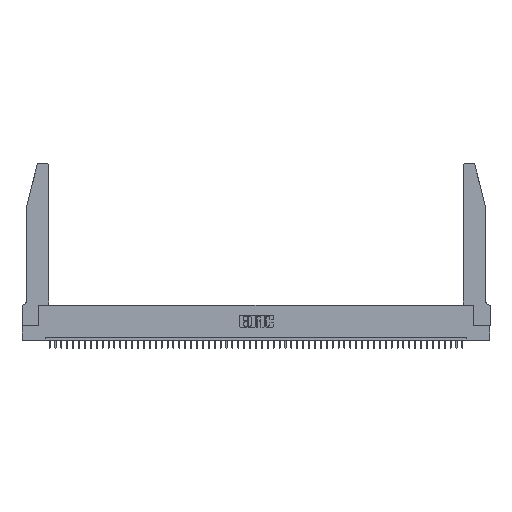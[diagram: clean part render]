
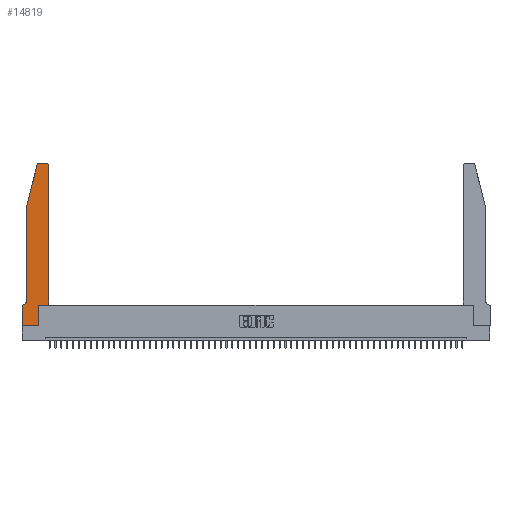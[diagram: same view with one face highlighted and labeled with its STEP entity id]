
A CAD part, top view. The second image highlights one B-rep face of the part: STEP entity #14819.
In plain terms, the highlighted planar face has unit normal (0, 0, 1).
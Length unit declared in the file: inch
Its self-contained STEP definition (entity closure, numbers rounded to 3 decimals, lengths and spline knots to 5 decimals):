
#916 = CIRCLE ( 'NONE', #51870, 0.07 ) ;
#919 = CARTESIAN_POINT ( 'NONE',  ( 0.0755, 2., 0.37 ) ) ;
#933 = DIRECTION ( 'NONE',  ( -1., 0., 0. ) ) ;
#1855 = VERTEX_POINT ( 'NONE', #25983 ) ;
#2791 = DIRECTION ( 'NONE',  ( -1., 0., 0. ) ) ;
#3752 = CARTESIAN_POINT ( 'NONE',  ( 0.2865, 0.35, 0.37 ) ) ;
#4103 = VECTOR ( 'NONE', #9275, 39.37008 ) ;
#4312 = EDGE_CURVE ( 'NONE', #38488, #1855, #916, .T. ) ;
#4542 = EDGE_LOOP ( 'NONE', ( #33524, #12257, #28069, #42367, #4695, #42255, #17631, #28983, #12638, #35962, #44566, #4682 ) ) ;
#4682 = ORIENTED_EDGE ( 'NONE', *, *, #17564, .T. ) ;
#4695 = ORIENTED_EDGE ( 'NONE', *, *, #4312, .T. ) ;
#5327 = LINE ( 'NONE', #21493, #29639 ) ;
#5565 = EDGE_CURVE ( 'NONE', #1855, #5975, #53952, .T. ) ;
#5975 = VERTEX_POINT ( 'NONE', #29071 ) ;
#6150 = VERTEX_POINT ( 'NONE', #25488 ) ;
#6459 = DIRECTION ( 'NONE',  ( 0., 0., 1. ) ) ;
#7187 = DIRECTION ( 'NONE',  ( -1., 0., 0. ) ) ;
#7304 = VERTEX_POINT ( 'NONE', #8736 ) ;
#7471 = CARTESIAN_POINT ( 'NONE',  ( 0., 0., 0.37 ) ) ;
#8736 = CARTESIAN_POINT ( 'NONE',  ( 0., 0., 0.37 ) ) ;
#9035 = EDGE_CURVE ( 'NONE', #6150, #38488, #21756, .T. ) ;
#9275 = DIRECTION ( 'NONE',  ( 0., 1., 0. ) ) ;
#10089 = CARTESIAN_POINT ( 'NONE',  ( 0.4505, 0.35, 0.37 ) ) ;
#11452 = VERTEX_POINT ( 'NONE', #41400 ) ;
#11808 = DIRECTION ( 'NONE',  ( 1., 0., 0. ) ) ;
#12257 = ORIENTED_EDGE ( 'NONE', *, *, #46270, .T. ) ;
#12519 = EDGE_CURVE ( 'NONE', #42337, #19759, #38734, .T. ) ;
#12638 = ORIENTED_EDGE ( 'NONE', *, *, #36609, .T. ) ;
#14085 = DIRECTION ( 'NONE',  ( -0.239, -0.971, 0. ) ) ;
#14819 = ADVANCED_FACE ( 'NONE', ( #31727 ), #40003, .T. ) ;
#14979 = CARTESIAN_POINT ( 'NONE',  ( 0.2865, 0., 0.37 ) ) ;
#15397 = CARTESIAN_POINT ( 'NONE',  ( 0.4205, 2.72, 0.37 ) ) ;
#15540 = CARTESIAN_POINT ( 'NONE',  ( 0.284, 2.72, 0.37 ) ) ;
#16439 = CARTESIAN_POINT ( 'NONE',  ( 0.4505, 0.35, 0.37 ) ) ;
#16645 = AXIS2_PLACEMENT_3D ( 'NONE', #15540, #44771, #53853 ) ;
#17564 = EDGE_CURVE ( 'NONE', #19759, #11452, #22466, .T. ) ;
#17631 = ORIENTED_EDGE ( 'NONE', *, *, #47384, .T. ) ;
#18322 = VECTOR ( 'NONE', #14085, 39.37008 ) ;
#19759 = VERTEX_POINT ( 'NONE', #34842 ) ;
#21493 = CARTESIAN_POINT ( 'NONE',  ( 0.2605, 2.75, 0.37 ) ) ;
#21756 = LINE ( 'NONE', #919, #53986 ) ;
#22039 = VERTEX_POINT ( 'NONE', #14979 ) ;
#22466 = CIRCLE ( 'NONE', #40937, 0.03 ) ;
#23005 = DIRECTION ( 'NONE',  ( 0., -1., 0. ) ) ;
#23827 = VERTEX_POINT ( 'NONE', #51852 ) ;
#23949 = LINE ( 'NONE', #7471, #35886 ) ;
#25007 = CARTESIAN_POINT ( 'NONE',  ( 0.0755, 0.35, 0.37 ) ) ;
#25386 = CARTESIAN_POINT ( 'NONE',  ( 0.25487, 2.72718, 0.37 ) ) ;
#25488 = CARTESIAN_POINT ( 'NONE',  ( 0.0755, 2., 0.37 ) ) ;
#25541 = DIRECTION ( 'NONE',  ( 1., 0., 0. ) ) ;
#25983 = CARTESIAN_POINT ( 'NONE',  ( 0.0055, 0.35, 0.37 ) ) ;
#26059 = LINE ( 'NONE', #38212, #48997 ) ;
#26320 = CARTESIAN_POINT ( 'NONE',  ( 0., 0., 0.37 ) ) ;
#26551 = CARTESIAN_POINT ( 'NONE',  ( 0.2865, 0.35, 0.37 ) ) ;
#28069 = ORIENTED_EDGE ( 'NONE', *, *, #40839, .T. ) ;
#28983 = ORIENTED_EDGE ( 'NONE', *, *, #45547, .T. ) ;
#29071 = CARTESIAN_POINT ( 'NONE',  ( 0., 0.35, 0.37 ) ) ;
#29639 = VECTOR ( 'NONE', #933, 39.37008 ) ;
#30005 = DIRECTION ( 'NONE',  ( 0., -1., 0. ) ) ;
#30893 = DIRECTION ( 'NONE',  ( 0., 0., 1. ) ) ;
#31727 = FACE_OUTER_BOUND ( 'NONE', #4542, .T. ) ;
#31800 = CARTESIAN_POINT ( 'NONE',  ( 0.0755, 0.42, 0.37 ) ) ;
#33524 = ORIENTED_EDGE ( 'NONE', *, *, #37567, .T. ) ;
#34842 = CARTESIAN_POINT ( 'NONE',  ( 0.4505, 2.72, 0.37 ) ) ;
#35886 = VECTOR ( 'NONE', #11808, 39.37008 ) ;
#35962 = ORIENTED_EDGE ( 'NONE', *, *, #44086, .T. ) ;
#36609 = EDGE_CURVE ( 'NONE', #22039, #54226, #39236, .T. ) ;
#37567 = EDGE_CURVE ( 'NONE', #11452, #23827, #5327, .T. ) ;
#37724 = CIRCLE ( 'NONE', #16645, 0.03 ) ;
#38212 = CARTESIAN_POINT ( 'NONE',  ( 0.4505, 0.35, 0.37 ) ) ;
#38488 = VERTEX_POINT ( 'NONE', #31800 ) ;
#38734 = LINE ( 'NONE', #16439, #4103 ) ;
#39236 = LINE ( 'NONE', #26551, #50699 ) ;
#40003 = PLANE ( 'NONE',  #44638 ) ;
#40839 = EDGE_CURVE ( 'NONE', #48117, #6150, #47966, .T. ) ;
#40937 = AXIS2_PLACEMENT_3D ( 'NONE', #15397, #30893, #44616 ) ;
#41363 = VECTOR ( 'NONE', #23005, 39.37008 ) ;
#41400 = CARTESIAN_POINT ( 'NONE',  ( 0.4205, 2.75, 0.37 ) ) ;
#42255 = ORIENTED_EDGE ( 'NONE', *, *, #5565, .T. ) ;
#42337 = VERTEX_POINT ( 'NONE', #10089 ) ;
#42367 = ORIENTED_EDGE ( 'NONE', *, *, #9035, .T. ) ;
#43395 = DIRECTION ( 'NONE',  ( 0., 1., 0. ) ) ;
#44086 = EDGE_CURVE ( 'NONE', #54226, #42337, #26059, .T. ) ;
#44566 = ORIENTED_EDGE ( 'NONE', *, *, #12519, .T. ) ;
#44588 = DIRECTION ( 'NONE',  ( 0., 0., -1. ) ) ;
#44616 = DIRECTION ( 'NONE',  ( 1., 0., 0. ) ) ;
#44638 = AXIS2_PLACEMENT_3D ( 'NONE', #49100, #6459, #53229 ) ;
#44771 = DIRECTION ( 'NONE',  ( 0., 0., 1. ) ) ;
#45547 = EDGE_CURVE ( 'NONE', #7304, #22039, #23949, .T. ) ;
#46270 = EDGE_CURVE ( 'NONE', #23827, #48117, #37724, .T. ) ;
#47384 = EDGE_CURVE ( 'NONE', #5975, #7304, #51658, .T. ) ;
#47966 = LINE ( 'NONE', #51540, #18322 ) ;
#48117 = VERTEX_POINT ( 'NONE', #25386 ) ;
#48163 = CARTESIAN_POINT ( 'NONE',  ( 0.0055, 0.42, 0.37 ) ) ;
#48997 = VECTOR ( 'NONE', #25541, 39.37008 ) ;
#49100 = CARTESIAN_POINT ( 'NONE',  ( 0., 0.35, 0.37 ) ) ;
#50699 = VECTOR ( 'NONE', #43395, 39.37008 ) ;
#51540 = CARTESIAN_POINT ( 'NONE',  ( 0.0755, 2., 0.37 ) ) ;
#51658 = LINE ( 'NONE', #26320, #41363 ) ;
#51852 = CARTESIAN_POINT ( 'NONE',  ( 0.284, 2.75, 0.37 ) ) ;
#51870 = AXIS2_PLACEMENT_3D ( 'NONE', #48163, #44588, #2791 ) ;
#51954 = VECTOR ( 'NONE', #7187, 39.37008 ) ;
#53229 = DIRECTION ( 'NONE',  ( 1., 0., 0. ) ) ;
#53853 = DIRECTION ( 'NONE',  ( 1., 0., 0. ) ) ;
#53952 = LINE ( 'NONE', #25007, #51954 ) ;
#53986 = VECTOR ( 'NONE', #30005, 39.37008 ) ;
#54226 = VERTEX_POINT ( 'NONE', #3752 ) ;
